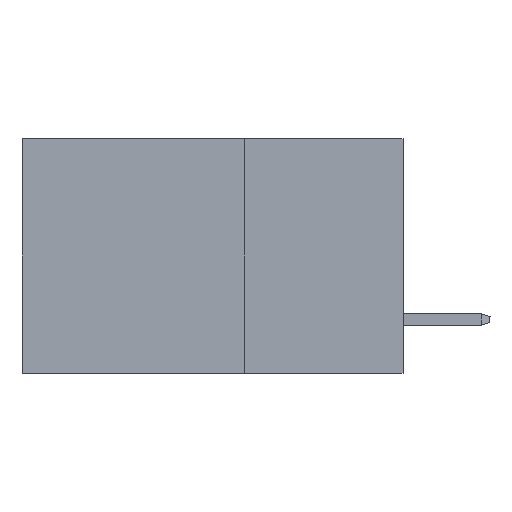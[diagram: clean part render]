
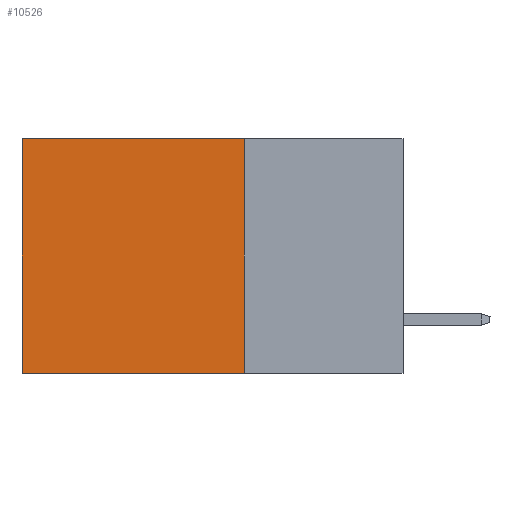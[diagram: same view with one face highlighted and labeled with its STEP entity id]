
A CAD part, left-side view. The second image highlights one B-rep face of the part: STEP entity #10526.
In plain terms, the highlighted planar face has unit normal (-1, 0, 0).
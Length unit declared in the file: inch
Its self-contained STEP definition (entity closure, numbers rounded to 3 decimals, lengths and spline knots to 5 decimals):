
#188 = CARTESIAN_POINT ( 'NONE',  ( 0.2875, 0.25, -0.37 ) ) ;
#4583 = VECTOR ( 'NONE', #24551, 39.37008 ) ;
#9870 = CARTESIAN_POINT ( 'NONE',  ( 0.2875, 0.25, 0. ) ) ;
#9991 = CARTESIAN_POINT ( 'NONE',  ( 0.2875, 0.6, -0.37 ) ) ;
#10032 = LINE ( 'NONE', #188, #10957 ) ;
#10037 = LINE ( 'NONE', #9870, #13583 ) ;
#10510 = ORIENTED_EDGE ( 'NONE', *, *, #31118, .F. ) ;
#10526 = ADVANCED_FACE ( 'NONE', ( #21919 ), #19430, .F. ) ;
#10738 = CARTESIAN_POINT ( 'NONE',  ( 0.2875, 0.25, 0. ) ) ;
#10957 = VECTOR ( 'NONE', #17694, 39.37008 ) ;
#12065 = LINE ( 'NONE', #17224, #4583 ) ;
#12220 = EDGE_LOOP ( 'NONE', ( #23495, #14089, #10510, #31517 ) ) ;
#12791 = EDGE_CURVE ( 'NONE', #32712, #25861, #10037, .T. ) ;
#13300 = CARTESIAN_POINT ( 'NONE',  ( 0.2875, 0.6, 0. ) ) ;
#13583 = VECTOR ( 'NONE', #22846, 39.37008 ) ;
#13787 = VECTOR ( 'NONE', #15223, 39.37008 ) ;
#13921 = CARTESIAN_POINT ( 'NONE',  ( 0.2875, 0.25, -0.37 ) ) ;
#14089 = ORIENTED_EDGE ( 'NONE', *, *, #27627, .F. ) ;
#14426 = DIRECTION ( 'NONE',  ( 0., 0., -1. ) ) ;
#14661 = EDGE_CURVE ( 'NONE', #25861, #17982, #12065, .T. ) ;
#15223 = DIRECTION ( 'NONE',  ( 0., 0., -1. ) ) ;
#16920 = DIRECTION ( 'NONE',  ( 1., 0., 0. ) ) ;
#17224 = CARTESIAN_POINT ( 'NONE',  ( 0.2875, 0.6, 0. ) ) ;
#17694 = DIRECTION ( 'NONE',  ( 0., 1., 0. ) ) ;
#17982 = VERTEX_POINT ( 'NONE', #9991 ) ;
#19430 = PLANE ( 'NONE',  #19981 ) ;
#19981 = AXIS2_PLACEMENT_3D ( 'NONE', #29596, #16920, #14426 ) ;
#21919 = FACE_OUTER_BOUND ( 'NONE', #12220, .T. ) ;
#22846 = DIRECTION ( 'NONE',  ( 0., 1., 0. ) ) ;
#23495 = ORIENTED_EDGE ( 'NONE', *, *, #14661, .T. ) ;
#24551 = DIRECTION ( 'NONE',  ( 0., 0., -1. ) ) ;
#25099 = VERTEX_POINT ( 'NONE', #13921 ) ;
#25861 = VERTEX_POINT ( 'NONE', #13300 ) ;
#27627 = EDGE_CURVE ( 'NONE', #25099, #17982, #10032, .T. ) ;
#28233 = LINE ( 'NONE', #10738, #13787 ) ;
#29596 = CARTESIAN_POINT ( 'NONE',  ( 0.2875, 0.25, 0. ) ) ;
#30215 = CARTESIAN_POINT ( 'NONE',  ( 0.2875, 0.25, 0. ) ) ;
#31118 = EDGE_CURVE ( 'NONE', #32712, #25099, #28233, .T. ) ;
#31517 = ORIENTED_EDGE ( 'NONE', *, *, #12791, .T. ) ;
#32712 = VERTEX_POINT ( 'NONE', #30215 ) ;
